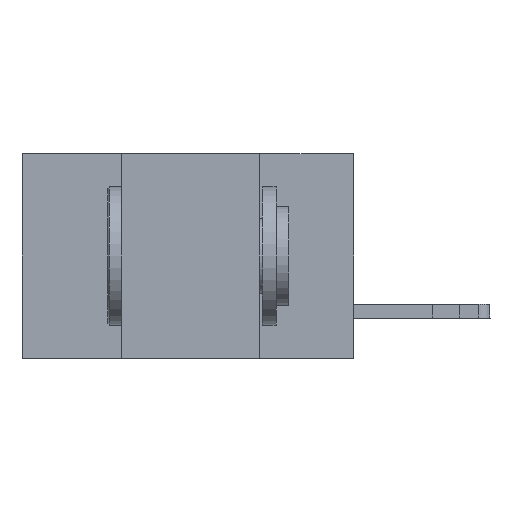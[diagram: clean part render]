
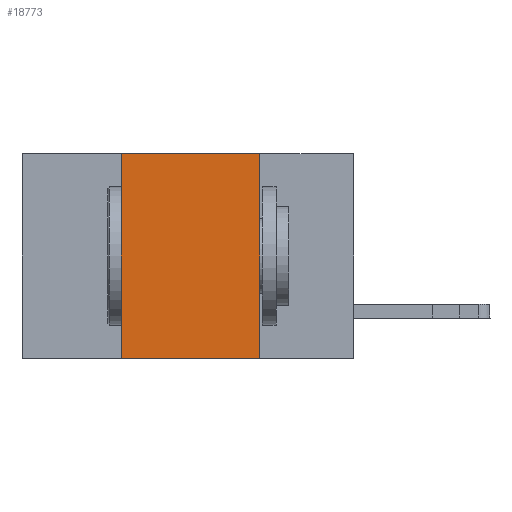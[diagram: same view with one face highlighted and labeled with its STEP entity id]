
A CAD part, left-side view. The second image highlights one B-rep face of the part: STEP entity #18773.
In plain terms, the highlighted planar face has unit normal (-1, 0, 0).
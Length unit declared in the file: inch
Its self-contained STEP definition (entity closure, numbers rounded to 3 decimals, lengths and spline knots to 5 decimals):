
#770 = CARTESIAN_POINT ( 'NONE',  ( 0., 0.42, 0. ) ) ;
#3054 = LINE ( 'NONE', #13913, #14817 ) ;
#4349 = DIRECTION ( 'NONE',  ( 0., -1., 0. ) ) ;
#4680 = EDGE_CURVE ( 'NONE', #22268, #4780, #9360, .T. ) ;
#4780 = VERTEX_POINT ( 'NONE', #15661 ) ;
#5528 = CARTESIAN_POINT ( 'NONE',  ( 0., 0.42, -0.37 ) ) ;
#7578 = EDGE_CURVE ( 'NONE', #14021, #15632, #22516, .T. ) ;
#7991 = LINE ( 'NONE', #770, #9627 ) ;
#8357 = FACE_OUTER_BOUND ( 'NONE', #12236, .T. ) ;
#9360 = LINE ( 'NONE', #13285, #17791 ) ;
#9422 = DIRECTION ( 'NONE',  ( 0., 0., 1. ) ) ;
#9627 = VECTOR ( 'NONE', #9422, 39.37008 ) ;
#11638 = AXIS2_PLACEMENT_3D ( 'NONE', #23076, #12287, #22957 ) ;
#12236 = EDGE_LOOP ( 'NONE', ( #15664, #12480, #20431, #21313 ) ) ;
#12287 = DIRECTION ( 'NONE',  ( 1., 0., 0. ) ) ;
#12480 = ORIENTED_EDGE ( 'NONE', *, *, #4680, .F. ) ;
#13285 = CARTESIAN_POINT ( 'NONE',  ( 0., 0.6, 0. ) ) ;
#13913 = CARTESIAN_POINT ( 'NONE',  ( 0., 0.17, 0. ) ) ;
#14021 = VERTEX_POINT ( 'NONE', #5528 ) ;
#14493 = EDGE_CURVE ( 'NONE', #14021, #22268, #7991, .T. ) ;
#14817 = VECTOR ( 'NONE', #19448, 39.37008 ) ;
#15068 = DIRECTION ( 'NONE',  ( 0., -1., 0. ) ) ;
#15632 = VERTEX_POINT ( 'NONE', #18413 ) ;
#15661 = CARTESIAN_POINT ( 'NONE',  ( 0., 0.17, 0. ) ) ;
#15664 = ORIENTED_EDGE ( 'NONE', *, *, #23087, .F. ) ;
#15925 = VECTOR ( 'NONE', #15068, 39.37008 ) ;
#17448 = PLANE ( 'NONE',  #11638 ) ;
#17791 = VECTOR ( 'NONE', #4349, 39.37008 ) ;
#18413 = CARTESIAN_POINT ( 'NONE',  ( 0., 0.17, -0.37 ) ) ;
#18773 = ADVANCED_FACE ( 'NONE', ( #8357 ), #17448, .F. ) ;
#19448 = DIRECTION ( 'NONE',  ( 0., 0., -1. ) ) ;
#20431 = ORIENTED_EDGE ( 'NONE', *, *, #14493, .F. ) ;
#20838 = CARTESIAN_POINT ( 'NONE',  ( 0., 0.6, -0.37 ) ) ;
#21313 = ORIENTED_EDGE ( 'NONE', *, *, #7578, .T. ) ;
#21527 = CARTESIAN_POINT ( 'NONE',  ( 0., 0.42, 0. ) ) ;
#22268 = VERTEX_POINT ( 'NONE', #21527 ) ;
#22516 = LINE ( 'NONE', #20838, #15925 ) ;
#22957 = DIRECTION ( 'NONE',  ( 0., 0., -1. ) ) ;
#23076 = CARTESIAN_POINT ( 'NONE',  ( 0., 0.6, 0. ) ) ;
#23087 = EDGE_CURVE ( 'NONE', #4780, #15632, #3054, .T. ) ;
